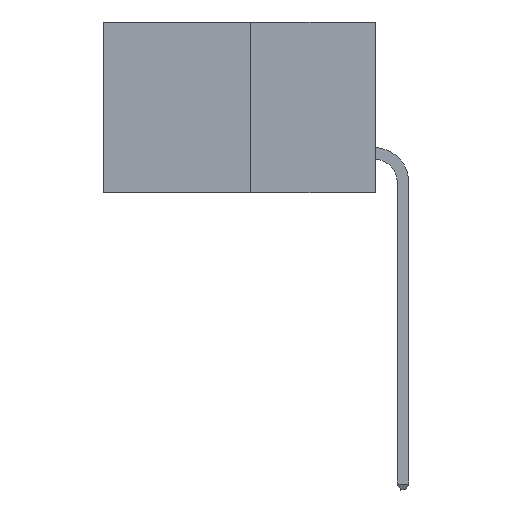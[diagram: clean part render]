
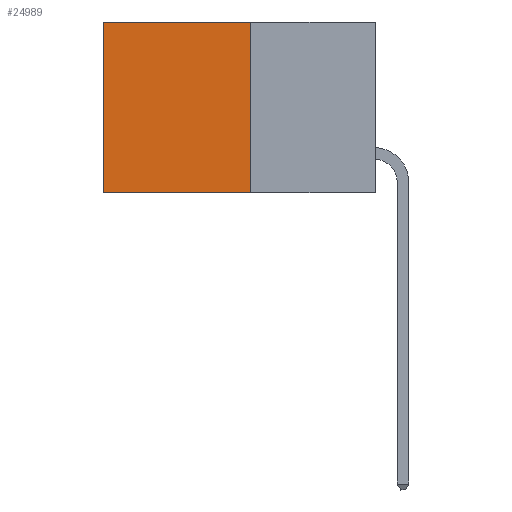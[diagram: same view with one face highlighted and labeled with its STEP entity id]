
A CAD part, left-side view. The second image highlights one B-rep face of the part: STEP entity #24989.
In plain terms, the highlighted planar face has unit normal (-1, 0, 0).
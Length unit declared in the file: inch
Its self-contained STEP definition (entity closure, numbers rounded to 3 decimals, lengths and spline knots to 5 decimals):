
#1058 = LINE ( 'NONE', #28313, #13627 ) ;
#2885 = VECTOR ( 'NONE', #29796, 39.37008 ) ;
#3056 = CARTESIAN_POINT ( 'NONE',  ( 0.277, 0.59, -0.37 ) ) ;
#4534 = FACE_OUTER_BOUND ( 'NONE', #13453, .T. ) ;
#5510 = CARTESIAN_POINT ( 'NONE',  ( 0.277, 0.27, -0.37 ) ) ;
#5630 = DIRECTION ( 'NONE',  ( 0., 0., -1. ) ) ;
#9631 = ORIENTED_EDGE ( 'NONE', *, *, #13215, .F. ) ;
#10292 = ORIENTED_EDGE ( 'NONE', *, *, #20234, .T. ) ;
#11063 = DIRECTION ( 'NONE',  ( 0., 0., -1. ) ) ;
#13130 = EDGE_CURVE ( 'NONE', #29691, #21466, #1058, .T. ) ;
#13215 = EDGE_CURVE ( 'NONE', #18572, #29691, #30622, .T. ) ;
#13453 = EDGE_LOOP ( 'NONE', ( #32185, #26557, #9631, #10292 ) ) ;
#13627 = VECTOR ( 'NONE', #30838, 39.37008 ) ;
#15611 = PLANE ( 'NONE',  #21726 ) ;
#15629 = LINE ( 'NONE', #3056, #22342 ) ;
#17146 = VECTOR ( 'NONE', #11063, 39.37008 ) ;
#18572 = VERTEX_POINT ( 'NONE', #19027 ) ;
#19027 = CARTESIAN_POINT ( 'NONE',  ( 0.277, 0.27, 0. ) ) ;
#20234 = EDGE_CURVE ( 'NONE', #18572, #22879, #29704, .T. ) ;
#20696 = DIRECTION ( 'NONE',  ( 1., 0., 0. ) ) ;
#21466 = VERTEX_POINT ( 'NONE', #27423 ) ;
#21726 = AXIS2_PLACEMENT_3D ( 'NONE', #5510, #20696, #5630 ) ;
#22342 = VECTOR ( 'NONE', #30720, 39.37008 ) ;
#22879 = VERTEX_POINT ( 'NONE', #32488 ) ;
#24989 = ADVANCED_FACE ( 'NONE', ( #4534 ), #15611, .F. ) ;
#26557 = ORIENTED_EDGE ( 'NONE', *, *, #13130, .F. ) ;
#27423 = CARTESIAN_POINT ( 'NONE',  ( 0.277, 0.59, -0.37 ) ) ;
#27877 = EDGE_CURVE ( 'NONE', #22879, #21466, #15629, .T. ) ;
#28313 = CARTESIAN_POINT ( 'NONE',  ( 0.277, 0.27, -0.37 ) ) ;
#29691 = VERTEX_POINT ( 'NONE', #31925 ) ;
#29704 = LINE ( 'NONE', #32181, #2885 ) ;
#29796 = DIRECTION ( 'NONE',  ( 0., 1., 0. ) ) ;
#30622 = LINE ( 'NONE', #31279, #17146 ) ;
#30720 = DIRECTION ( 'NONE',  ( 0., 0., -1. ) ) ;
#30838 = DIRECTION ( 'NONE',  ( 0., 1., 0. ) ) ;
#31279 = CARTESIAN_POINT ( 'NONE',  ( 0.277, 0.27, -0.37 ) ) ;
#31925 = CARTESIAN_POINT ( 'NONE',  ( 0.277, 0.27, -0.37 ) ) ;
#32181 = CARTESIAN_POINT ( 'NONE',  ( 0.277, 0.27, 0. ) ) ;
#32185 = ORIENTED_EDGE ( 'NONE', *, *, #27877, .T. ) ;
#32488 = CARTESIAN_POINT ( 'NONE',  ( 0.277, 0.59, 0. ) ) ;
